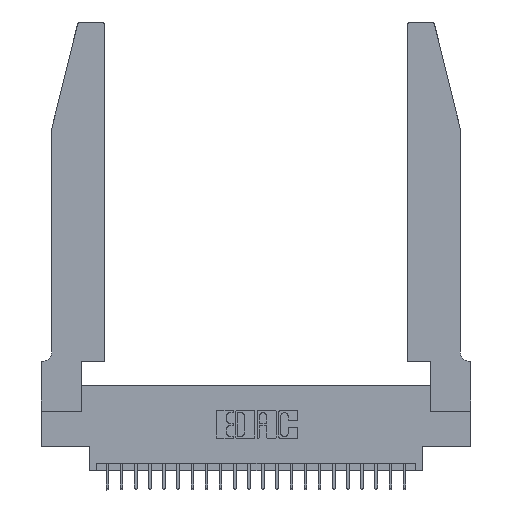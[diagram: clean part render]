
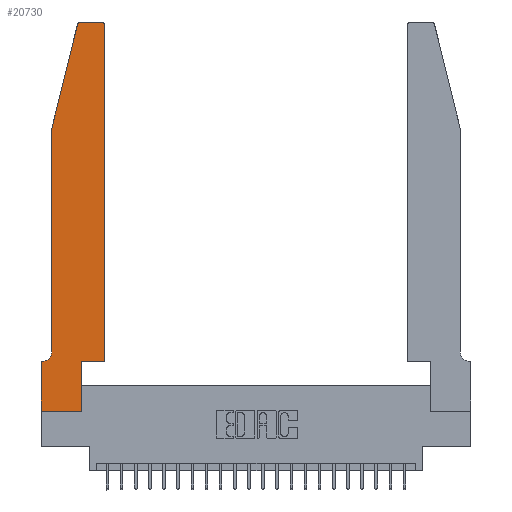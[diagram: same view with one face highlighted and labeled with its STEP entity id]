
A CAD part, top view. The second image highlights one B-rep face of the part: STEP entity #20730.
In plain terms, the highlighted planar face has unit normal (0, 0, 1).
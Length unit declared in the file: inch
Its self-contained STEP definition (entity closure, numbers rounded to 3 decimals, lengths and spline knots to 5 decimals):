
#30 = ORIENTED_EDGE ( 'NONE', *, *, #114, .T. ) ;
#114 = EDGE_CURVE ( 'NONE', #15799, #21196, #1444, .T. ) ;
#219 = DIRECTION ( 'NONE',  ( 0., 1., 0. ) ) ;
#505 = CARTESIAN_POINT ( 'NONE',  ( 0.0755, 0.35, 0.37 ) ) ;
#667 = EDGE_LOOP ( 'NONE', ( #23676, #1227, #15742, #23418, #13075, #16416, #30, #12910, #14993, #24245, #1196, #2574 ) ) ;
#1196 = ORIENTED_EDGE ( 'NONE', *, *, #2826, .T. ) ;
#1227 = ORIENTED_EDGE ( 'NONE', *, *, #12216, .T. ) ;
#1444 = LINE ( 'NONE', #3361, #22267 ) ;
#1893 = CARTESIAN_POINT ( 'NONE',  ( 0.4505, 0.35, 0.37 ) ) ;
#1967 = DIRECTION ( 'NONE',  ( 1., 0., 0. ) ) ;
#2574 = ORIENTED_EDGE ( 'NONE', *, *, #15459, .T. ) ;
#2783 = LINE ( 'NONE', #505, #18489 ) ;
#2826 = EDGE_CURVE ( 'NONE', #17119, #5762, #5549, .T. ) ;
#2887 = CIRCLE ( 'NONE', #17011, 0.07 ) ;
#3290 = CARTESIAN_POINT ( 'NONE',  ( 0.2865, 0.35, 0.37 ) ) ;
#3361 = CARTESIAN_POINT ( 'NONE',  ( 0., 0., 0.37 ) ) ;
#3517 = DIRECTION ( 'NONE',  ( 1., 0., 0. ) ) ;
#3596 = CARTESIAN_POINT ( 'NONE',  ( 0.2605, 2.75, 0.37 ) ) ;
#3785 = DIRECTION ( 'NONE',  ( 0., -1., 0. ) ) ;
#3791 = EDGE_CURVE ( 'NONE', #11238, #23600, #24478, .T. ) ;
#3893 = AXIS2_PLACEMENT_3D ( 'NONE', #5290, #13120, #3517 ) ;
#4326 = DIRECTION ( 'NONE',  ( -1., 0., 0. ) ) ;
#5290 = CARTESIAN_POINT ( 'NONE',  ( 0.4205, 2.72, 0.37 ) ) ;
#5534 = LINE ( 'NONE', #24585, #13143 ) ;
#5549 = LINE ( 'NONE', #21214, #7319 ) ;
#5583 = LINE ( 'NONE', #1893, #18308 ) ;
#5762 = VERTEX_POINT ( 'NONE', #8244 ) ;
#5869 = CARTESIAN_POINT ( 'NONE',  ( 0.284, 2.75, 0.37 ) ) ;
#6029 = CARTESIAN_POINT ( 'NONE',  ( 0.284, 2.72, 0.37 ) ) ;
#6096 = EDGE_CURVE ( 'NONE', #20578, #12646, #11617, .T. ) ;
#6261 = DIRECTION ( 'NONE',  ( 1., 0., 0. ) ) ;
#6278 = CIRCLE ( 'NONE', #9513, 0.03 ) ;
#7319 = VECTOR ( 'NONE', #18944, 39.37008 ) ;
#8244 = CARTESIAN_POINT ( 'NONE',  ( 0.4505, 2.72, 0.37 ) ) ;
#8286 = EDGE_CURVE ( 'NONE', #12646, #17119, #5583, .T. ) ;
#9513 = AXIS2_PLACEMENT_3D ( 'NONE', #6029, #23556, #1967 ) ;
#9536 = VECTOR ( 'NONE', #219, 39.37008 ) ;
#10923 = EDGE_CURVE ( 'NONE', #21196, #20578, #22519, .T. ) ;
#11058 = DIRECTION ( 'NONE',  ( -1., 0., 0. ) ) ;
#11237 = DIRECTION ( 'NONE',  ( -0.239, -0.971, 0. ) ) ;
#11238 = VERTEX_POINT ( 'NONE', #20958 ) ;
#11287 = DIRECTION ( 'NONE',  ( 1., 0., 0. ) ) ;
#11343 = DIRECTION ( 'NONE',  ( 0., -1., 0. ) ) ;
#11617 = LINE ( 'NONE', #23335, #9536 ) ;
#12136 = EDGE_CURVE ( 'NONE', #22968, #11238, #5534, .T. ) ;
#12216 = EDGE_CURVE ( 'NONE', #18192, #22968, #6278, .T. ) ;
#12583 = CARTESIAN_POINT ( 'NONE',  ( 0.0755, 0.42, 0.37 ) ) ;
#12585 = CARTESIAN_POINT ( 'NONE',  ( 0.4205, 2.75, 0.37 ) ) ;
#12646 = VERTEX_POINT ( 'NONE', #3290 ) ;
#12773 = CARTESIAN_POINT ( 'NONE',  ( 0., 0., 0.37 ) ) ;
#12910 = ORIENTED_EDGE ( 'NONE', *, *, #10923, .T. ) ;
#13075 = ORIENTED_EDGE ( 'NONE', *, *, #23742, .T. ) ;
#13120 = DIRECTION ( 'NONE',  ( 0., 0., 1. ) ) ;
#13143 = VECTOR ( 'NONE', #11237, 39.37008 ) ;
#14774 = CIRCLE ( 'NONE', #3893, 0.03 ) ;
#14837 = CARTESIAN_POINT ( 'NONE',  ( 0., 0.35, 0.37 ) ) ;
#14961 = LINE ( 'NONE', #3596, #21395 ) ;
#14993 = ORIENTED_EDGE ( 'NONE', *, *, #6096, .T. ) ;
#15459 = EDGE_CURVE ( 'NONE', #5762, #15813, #14774, .T. ) ;
#15497 = VECTOR ( 'NONE', #11287, 39.37008 ) ;
#15742 = ORIENTED_EDGE ( 'NONE', *, *, #12136, .T. ) ;
#15799 = VERTEX_POINT ( 'NONE', #14837 ) ;
#15813 = VERTEX_POINT ( 'NONE', #12585 ) ;
#15858 = CARTESIAN_POINT ( 'NONE',  ( 0., 0.35, 0.37 ) ) ;
#16416 = ORIENTED_EDGE ( 'NONE', *, *, #16816, .T. ) ;
#16816 = EDGE_CURVE ( 'NONE', #19122, #15799, #2783, .T. ) ;
#16853 = DIRECTION ( 'NONE',  ( -1., 0., 0. ) ) ;
#17011 = AXIS2_PLACEMENT_3D ( 'NONE', #20530, #20789, #16853 ) ;
#17119 = VERTEX_POINT ( 'NONE', #17434 ) ;
#17434 = CARTESIAN_POINT ( 'NONE',  ( 0.4505, 0.35, 0.37 ) ) ;
#17615 = PLANE ( 'NONE',  #20153 ) ;
#18192 = VERTEX_POINT ( 'NONE', #5869 ) ;
#18308 = VECTOR ( 'NONE', #24750, 39.37008 ) ;
#18489 = VECTOR ( 'NONE', #4326, 39.37008 ) ;
#18944 = DIRECTION ( 'NONE',  ( 0., 1., 0. ) ) ;
#18952 = CARTESIAN_POINT ( 'NONE',  ( 0.0755, 2., 0.37 ) ) ;
#19122 = VERTEX_POINT ( 'NONE', #19826 ) ;
#19530 = DIRECTION ( 'NONE',  ( 0., 0., 1. ) ) ;
#19754 = EDGE_CURVE ( 'NONE', #15813, #18192, #14961, .T. ) ;
#19826 = CARTESIAN_POINT ( 'NONE',  ( 0.0055, 0.35, 0.37 ) ) ;
#20153 = AXIS2_PLACEMENT_3D ( 'NONE', #15858, #19530, #6261 ) ;
#20530 = CARTESIAN_POINT ( 'NONE',  ( 0.0055, 0.42, 0.37 ) ) ;
#20578 = VERTEX_POINT ( 'NONE', #23295 ) ;
#20730 = ADVANCED_FACE ( 'NONE', ( #23796 ), #17615, .T. ) ;
#20789 = DIRECTION ( 'NONE',  ( 0., 0., -1. ) ) ;
#20958 = CARTESIAN_POINT ( 'NONE',  ( 0.0755, 2., 0.37 ) ) ;
#21196 = VERTEX_POINT ( 'NONE', #22658 ) ;
#21214 = CARTESIAN_POINT ( 'NONE',  ( 0.4505, 0.35, 0.37 ) ) ;
#21395 = VECTOR ( 'NONE', #11058, 39.37008 ) ;
#22267 = VECTOR ( 'NONE', #11343, 39.37008 ) ;
#22519 = LINE ( 'NONE', #12773, #15497 ) ;
#22658 = CARTESIAN_POINT ( 'NONE',  ( 0., 0., 0.37 ) ) ;
#22968 = VERTEX_POINT ( 'NONE', #24730 ) ;
#23295 = CARTESIAN_POINT ( 'NONE',  ( 0.2865, 0., 0.37 ) ) ;
#23321 = VECTOR ( 'NONE', #3785, 39.37008 ) ;
#23335 = CARTESIAN_POINT ( 'NONE',  ( 0.2865, 0.35, 0.37 ) ) ;
#23418 = ORIENTED_EDGE ( 'NONE', *, *, #3791, .T. ) ;
#23556 = DIRECTION ( 'NONE',  ( 0., 0., 1. ) ) ;
#23600 = VERTEX_POINT ( 'NONE', #12583 ) ;
#23676 = ORIENTED_EDGE ( 'NONE', *, *, #19754, .T. ) ;
#23742 = EDGE_CURVE ( 'NONE', #23600, #19122, #2887, .T. ) ;
#23796 = FACE_OUTER_BOUND ( 'NONE', #667, .T. ) ;
#24245 = ORIENTED_EDGE ( 'NONE', *, *, #8286, .T. ) ;
#24478 = LINE ( 'NONE', #18952, #23321 ) ;
#24585 = CARTESIAN_POINT ( 'NONE',  ( 0.0755, 2., 0.37 ) ) ;
#24730 = CARTESIAN_POINT ( 'NONE',  ( 0.25487, 2.72718, 0.37 ) ) ;
#24750 = DIRECTION ( 'NONE',  ( 1., 0., 0. ) ) ;
